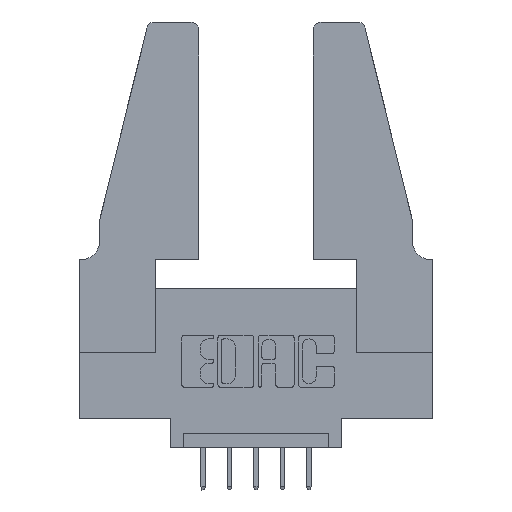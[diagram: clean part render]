
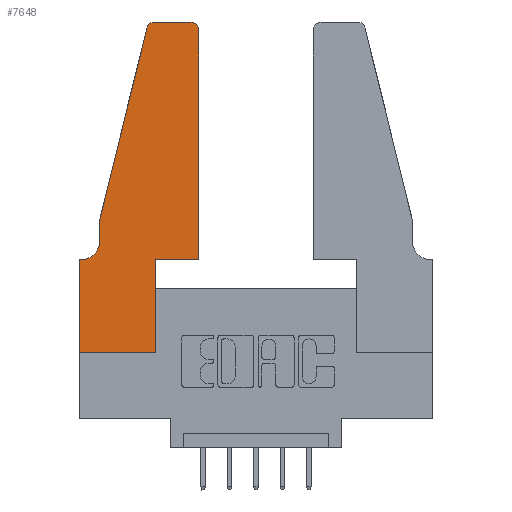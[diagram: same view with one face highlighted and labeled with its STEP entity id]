
A CAD part, top view. The second image highlights one B-rep face of the part: STEP entity #7648.
In plain terms, the highlighted planar face has unit normal (0, 0, 1).
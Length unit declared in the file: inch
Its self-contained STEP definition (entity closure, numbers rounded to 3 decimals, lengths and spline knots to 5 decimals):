
#102 = ORIENTED_EDGE ( 'NONE', *, *, #8733, .T. ) ;
#187 = VERTEX_POINT ( 'NONE', #4655 ) ;
#293 = DIRECTION ( 'NONE',  ( 0., 0., 1. ) ) ;
#458 = CARTESIAN_POINT ( 'NONE',  ( 0.0755, 0.5, 0.37 ) ) ;
#995 = EDGE_CURVE ( 'NONE', #2650, #187, #7591, .T. ) ;
#1096 = VERTEX_POINT ( 'NONE', #7390 ) ;
#1186 = DIRECTION ( 'NONE',  ( 0., 0., -1. ) ) ;
#1203 = CARTESIAN_POINT ( 'NONE',  ( 0.2865, 0.35, 0.37 ) ) ;
#1268 = DIRECTION ( 'NONE',  ( -1., 0., 0. ) ) ;
#1284 = CARTESIAN_POINT ( 'NONE',  ( 0.4205, 1.22, 0.37 ) ) ;
#1318 = CARTESIAN_POINT ( 'NONE',  ( 0., 0.35, 0.37 ) ) ;
#1342 = DIRECTION ( 'NONE',  ( -1., 0., 0. ) ) ;
#1346 = DIRECTION ( 'NONE',  ( -1., 0., 0. ) ) ;
#1376 = CARTESIAN_POINT ( 'NONE',  ( 0.4505, 0.35, 0.37 ) ) ;
#1826 = VECTOR ( 'NONE', #1346, 39.37008 ) ;
#1842 = DIRECTION ( 'NONE',  ( 0., 1., 0. ) ) ;
#2071 = ORIENTED_EDGE ( 'NONE', *, *, #2451, .T. ) ;
#2252 = DIRECTION ( 'NONE',  ( 0., 1., 0. ) ) ;
#2451 = EDGE_CURVE ( 'NONE', #11111, #2861, #8835, .T. ) ;
#2472 = ORIENTED_EDGE ( 'NONE', *, *, #10155, .T. ) ;
#2590 = EDGE_CURVE ( 'NONE', #2861, #2650, #8697, .T. ) ;
#2650 = VERTEX_POINT ( 'NONE', #8470 ) ;
#2731 = AXIS2_PLACEMENT_3D ( 'NONE', #1284, #8992, #4688 ) ;
#2760 = LINE ( 'NONE', #9959, #1826 ) ;
#2861 = VERTEX_POINT ( 'NONE', #458 ) ;
#2912 = ORIENTED_EDGE ( 'NONE', *, *, #4826, .T. ) ;
#2954 = ORIENTED_EDGE ( 'NONE', *, *, #995, .T. ) ;
#2960 = VERTEX_POINT ( 'NONE', #1203 ) ;
#2967 = VECTOR ( 'NONE', #7893, 39.37008 ) ;
#3020 = CARTESIAN_POINT ( 'NONE',  ( 0.4205, 1.25, 0.37 ) ) ;
#3517 = AXIS2_PLACEMENT_3D ( 'NONE', #8903, #293, #6275 ) ;
#3691 = VECTOR ( 'NONE', #1342, 39.37008 ) ;
#3806 = VECTOR ( 'NONE', #4359, 39.37008 ) ;
#3812 = CARTESIAN_POINT ( 'NONE',  ( 0.284, 1.25, 0.37 ) ) ;
#3843 = LINE ( 'NONE', #1376, #10000 ) ;
#3939 = CIRCLE ( 'NONE', #3517, 0.03 ) ;
#4101 = LINE ( 'NONE', #6458, #3691 ) ;
#4158 = VECTOR ( 'NONE', #8407, 39.37008 ) ;
#4178 = VERTEX_POINT ( 'NONE', #7124 ) ;
#4359 = DIRECTION ( 'NONE',  ( 1., 0., 0. ) ) ;
#4507 = ORIENTED_EDGE ( 'NONE', *, *, #5967, .T. ) ;
#4649 = CARTESIAN_POINT ( 'NONE',  ( 0.25487, 1.22718, 0.37 ) ) ;
#4655 = CARTESIAN_POINT ( 'NONE',  ( 0.0055, 0.35, 0.37 ) ) ;
#4684 = DIRECTION ( 'NONE',  ( 1., 0., 0. ) ) ;
#4688 = DIRECTION ( 'NONE',  ( 1., 0., 0. ) ) ;
#4821 = CARTESIAN_POINT ( 'NONE',  ( 0., 0., 0.37 ) ) ;
#4826 = EDGE_CURVE ( 'NONE', #6988, #2960, #10278, .T. ) ;
#4845 = ORIENTED_EDGE ( 'NONE', *, *, #9754, .T. ) ;
#5104 = CARTESIAN_POINT ( 'NONE',  ( 0., 0., 0.37 ) ) ;
#5330 = FACE_OUTER_BOUND ( 'NONE', #6588, .T. ) ;
#5456 = CARTESIAN_POINT ( 'NONE',  ( 0.0055, 0.42, 0.37 ) ) ;
#5799 = AXIS2_PLACEMENT_3D ( 'NONE', #5456, #1186, #1268 ) ;
#5934 = EDGE_CURVE ( 'NONE', #9259, #6375, #4101, .T. ) ;
#5965 = VECTOR ( 'NONE', #6420, 39.37008 ) ;
#5967 = EDGE_CURVE ( 'NONE', #8330, #6988, #9460, .T. ) ;
#6052 = CARTESIAN_POINT ( 'NONE',  ( 0., 0., 0.37 ) ) ;
#6275 = DIRECTION ( 'NONE',  ( 1., 0., 0. ) ) ;
#6375 = VERTEX_POINT ( 'NONE', #3812 ) ;
#6420 = DIRECTION ( 'NONE',  ( 1., 0., 0. ) ) ;
#6458 = CARTESIAN_POINT ( 'NONE',  ( 0.2605, 1.25, 0.37 ) ) ;
#6488 = AXIS2_PLACEMENT_3D ( 'NONE', #1318, #9026, #4684 ) ;
#6496 = ORIENTED_EDGE ( 'NONE', *, *, #9228, .T. ) ;
#6514 = PLANE ( 'NONE',  #6488 ) ;
#6588 = EDGE_LOOP ( 'NONE', ( #10462, #4845, #2071, #11008, #2954, #9315, #9668, #4507, #2912, #2472, #102, #6496 ) ) ;
#6912 = CARTESIAN_POINT ( 'NONE',  ( 0.2865, 0.35, 0.37 ) ) ;
#6988 = VERTEX_POINT ( 'NONE', #10506 ) ;
#7124 = CARTESIAN_POINT ( 'NONE',  ( 0.4505, 1.22, 0.37 ) ) ;
#7390 = CARTESIAN_POINT ( 'NONE',  ( 0.4505, 0.35, 0.37 ) ) ;
#7402 = LINE ( 'NONE', #5104, #9428 ) ;
#7591 = CIRCLE ( 'NONE', #5799, 0.07 ) ;
#7648 = ADVANCED_FACE ( 'NONE', ( #5330 ), #6514, .T. ) ;
#7893 = DIRECTION ( 'NONE',  ( -0.239, -0.971, 0. ) ) ;
#7991 = VECTOR ( 'NONE', #1842, 39.37008 ) ;
#8330 = VERTEX_POINT ( 'NONE', #6052 ) ;
#8407 = DIRECTION ( 'NONE',  ( 0., -1., 0. ) ) ;
#8470 = CARTESIAN_POINT ( 'NONE',  ( 0.0755, 0.42, 0.37 ) ) ;
#8697 = LINE ( 'NONE', #9307, #4158 ) ;
#8732 = VERTEX_POINT ( 'NONE', #9049 ) ;
#8733 = EDGE_CURVE ( 'NONE', #1096, #4178, #3843, .T. ) ;
#8835 = LINE ( 'NONE', #9742, #2967 ) ;
#8903 = CARTESIAN_POINT ( 'NONE',  ( 0.284, 1.22, 0.37 ) ) ;
#8992 = DIRECTION ( 'NONE',  ( 0., 0., 1. ) ) ;
#9026 = DIRECTION ( 'NONE',  ( 0., 0., 1. ) ) ;
#9049 = CARTESIAN_POINT ( 'NONE',  ( 0., 0.35, 0.37 ) ) ;
#9053 = CIRCLE ( 'NONE', #2731, 0.03 ) ;
#9228 = EDGE_CURVE ( 'NONE', #4178, #9259, #9053, .T. ) ;
#9259 = VERTEX_POINT ( 'NONE', #3020 ) ;
#9307 = CARTESIAN_POINT ( 'NONE',  ( 0.0755, 0.5, 0.37 ) ) ;
#9315 = ORIENTED_EDGE ( 'NONE', *, *, #9933, .T. ) ;
#9428 = VECTOR ( 'NONE', #10280, 39.37008 ) ;
#9460 = LINE ( 'NONE', #4821, #5965 ) ;
#9668 = ORIENTED_EDGE ( 'NONE', *, *, #10308, .T. ) ;
#9742 = CARTESIAN_POINT ( 'NONE',  ( 0.0755, 0.5, 0.37 ) ) ;
#9754 = EDGE_CURVE ( 'NONE', #6375, #11111, #3939, .T. ) ;
#9933 = EDGE_CURVE ( 'NONE', #187, #8732, #2760, .T. ) ;
#9959 = CARTESIAN_POINT ( 'NONE',  ( 0.0755, 0.35, 0.37 ) ) ;
#10000 = VECTOR ( 'NONE', #2252, 39.37008 ) ;
#10155 = EDGE_CURVE ( 'NONE', #2960, #1096, #10233, .T. ) ;
#10233 = LINE ( 'NONE', #10375, #3806 ) ;
#10278 = LINE ( 'NONE', #6912, #7991 ) ;
#10280 = DIRECTION ( 'NONE',  ( 0., -1., 0. ) ) ;
#10308 = EDGE_CURVE ( 'NONE', #8732, #8330, #7402, .T. ) ;
#10375 = CARTESIAN_POINT ( 'NONE',  ( 0.4505, 0.35, 0.37 ) ) ;
#10462 = ORIENTED_EDGE ( 'NONE', *, *, #5934, .T. ) ;
#10506 = CARTESIAN_POINT ( 'NONE',  ( 0.2865, 0., 0.37 ) ) ;
#11008 = ORIENTED_EDGE ( 'NONE', *, *, #2590, .T. ) ;
#11111 = VERTEX_POINT ( 'NONE', #4649 ) ;
